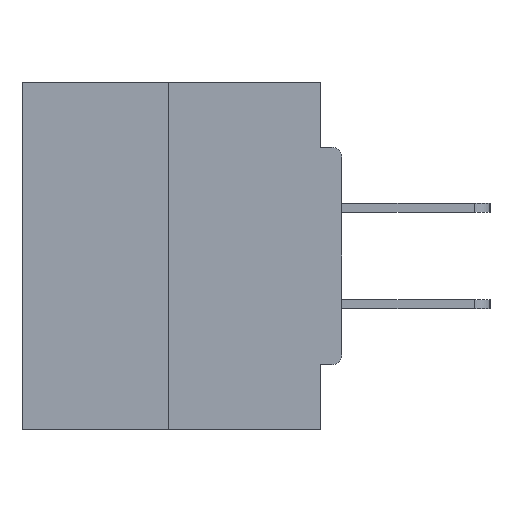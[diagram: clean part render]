
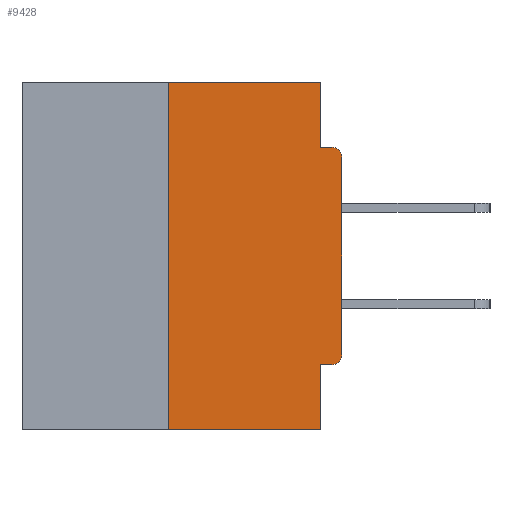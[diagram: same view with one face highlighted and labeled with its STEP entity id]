
A CAD part, left-side view. The second image highlights one B-rep face of the part: STEP entity #9428.
In plain terms, the highlighted planar face has unit normal (-1, 0, 0).
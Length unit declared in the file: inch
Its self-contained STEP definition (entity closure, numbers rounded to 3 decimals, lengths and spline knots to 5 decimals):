
#178 = LINE ( 'NONE', #2677, #25718 ) ;
#254 = PLANE ( 'NONE',  #14358 ) ;
#578 = CARTESIAN_POINT ( 'NONE',  ( 0., 0., -0.1085 ) ) ;
#690 = DIRECTION ( 'NONE',  ( 0., -1., 0. ) ) ;
#1343 = ORIENTED_EDGE ( 'NONE', *, *, #20671, .T. ) ;
#1772 = EDGE_CURVE ( 'NONE', #17126, #13864, #31024, .T. ) ;
#2656 = VECTOR ( 'NONE', #16002, 39.37008 ) ;
#2677 = CARTESIAN_POINT ( 'NONE',  ( 0., 0., -0.4065 ) ) ;
#2802 = VECTOR ( 'NONE', #17738, 39.37008 ) ;
#4215 = DIRECTION ( 'NONE',  ( 1., 0., 0. ) ) ;
#4961 = EDGE_CURVE ( 'NONE', #32058, #18116, #178, .T. ) ;
#5368 = VERTEX_POINT ( 'NONE', #33887 ) ;
#5515 = VERTEX_POINT ( 'NONE', #578 ) ;
#6188 = DIRECTION ( 'NONE',  ( 0., -1., 0. ) ) ;
#6482 = DIRECTION ( 'NONE',  ( 0., 0., -1. ) ) ;
#6739 = CARTESIAN_POINT ( 'NONE',  ( 0., 0.031, -0.5 ) ) ;
#7524 = LINE ( 'NONE', #21823, #31337 ) ;
#8227 = ORIENTED_EDGE ( 'NONE', *, *, #1772, .F. ) ;
#8964 = CARTESIAN_POINT ( 'NONE',  ( 0., 0.015, -0.1085 ) ) ;
#9094 = CARTESIAN_POINT ( 'NONE',  ( 0., 0., -0.0935 ) ) ;
#9354 = EDGE_CURVE ( 'NONE', #13864, #20374, #30465, .T. ) ;
#9428 = ADVANCED_FACE ( 'NONE', ( #26190 ), #254, .F. ) ;
#9786 = ORIENTED_EDGE ( 'NONE', *, *, #19300, .T. ) ;
#10267 = ORIENTED_EDGE ( 'NONE', *, *, #32802, .T. ) ;
#10586 = CARTESIAN_POINT ( 'NONE',  ( 0., 0.25, -0.5 ) ) ;
#10591 = VECTOR ( 'NONE', #6188, 39.37008 ) ;
#10795 = CIRCLE ( 'NONE', #32243, 0.015 ) ;
#11548 = LINE ( 'NONE', #18531, #13664 ) ;
#11606 = DIRECTION ( 'NONE',  ( 0., -1., 0. ) ) ;
#13664 = VECTOR ( 'NONE', #32955, 39.37008 ) ;
#13775 = CARTESIAN_POINT ( 'NONE',  ( 0., 0.25, 0. ) ) ;
#13864 = VERTEX_POINT ( 'NONE', #21802 ) ;
#14011 = CARTESIAN_POINT ( 'NONE',  ( 0., 0.015, -0.3915 ) ) ;
#14358 = AXIS2_PLACEMENT_3D ( 'NONE', #32922, #4215, #6482 ) ;
#14621 = EDGE_LOOP ( 'NONE', ( #8227, #24536, #34592, #26062, #24534, #9786, #1343, #10267, #15903, #28157 ) ) ;
#15578 = VERTEX_POINT ( 'NONE', #10586 ) ;
#15903 = ORIENTED_EDGE ( 'NONE', *, *, #22253, .F. ) ;
#16002 = DIRECTION ( 'NONE',  ( 0., 0., 1. ) ) ;
#16354 = CARTESIAN_POINT ( 'NONE',  ( 0., 0.25, 0. ) ) ;
#16833 = EDGE_CURVE ( 'NONE', #15578, #17126, #29869, .T. ) ;
#17126 = VERTEX_POINT ( 'NONE', #13775 ) ;
#17738 = DIRECTION ( 'NONE',  ( 0., 0., -1. ) ) ;
#18116 = VERTEX_POINT ( 'NONE', #33922 ) ;
#18531 = CARTESIAN_POINT ( 'NONE',  ( 0., 0., 0. ) ) ;
#19300 = EDGE_CURVE ( 'NONE', #32058, #5368, #10795, .T. ) ;
#19548 = CARTESIAN_POINT ( 'NONE',  ( 0., 0.015, -0.4065 ) ) ;
#19780 = CARTESIAN_POINT ( 'NONE',  ( 0., 0.46, 0. ) ) ;
#20374 = VERTEX_POINT ( 'NONE', #23149 ) ;
#20671 = EDGE_CURVE ( 'NONE', #5368, #5515, #11548, .T. ) ;
#21745 = DIRECTION ( 'NONE',  ( 0., 1., 0. ) ) ;
#21802 = CARTESIAN_POINT ( 'NONE',  ( 0., 0.031, 0. ) ) ;
#21823 = CARTESIAN_POINT ( 'NONE',  ( 0., 0.031, -0.5 ) ) ;
#22253 = EDGE_CURVE ( 'NONE', #20374, #32228, #28011, .T. ) ;
#22376 = CARTESIAN_POINT ( 'NONE',  ( 0., 0.46, -0.5 ) ) ;
#22562 = DIRECTION ( 'NONE',  ( 0., 0., -1. ) ) ;
#22721 = EDGE_CURVE ( 'NONE', #18116, #33283, #7524, .T. ) ;
#23149 = CARTESIAN_POINT ( 'NONE',  ( 0., 0.031, -0.0935 ) ) ;
#23221 = EDGE_CURVE ( 'NONE', #15578, #33283, #33869, .T. ) ;
#24534 = ORIENTED_EDGE ( 'NONE', *, *, #4961, .F. ) ;
#24536 = ORIENTED_EDGE ( 'NONE', *, *, #16833, .F. ) ;
#25058 = VECTOR ( 'NONE', #11606, 39.37008 ) ;
#25718 = VECTOR ( 'NONE', #21745, 39.37008 ) ;
#25752 = CIRCLE ( 'NONE', #32561, 0.015 ) ;
#26062 = ORIENTED_EDGE ( 'NONE', *, *, #22721, .F. ) ;
#26190 = FACE_OUTER_BOUND ( 'NONE', #14621, .T. ) ;
#26635 = DIRECTION ( 'NONE',  ( 0., 0., -1. ) ) ;
#28011 = LINE ( 'NONE', #9094, #25058 ) ;
#28157 = ORIENTED_EDGE ( 'NONE', *, *, #9354, .F. ) ;
#29869 = LINE ( 'NONE', #16354, #2656 ) ;
#30343 = DIRECTION ( 'NONE',  ( -1., 0., 0. ) ) ;
#30465 = LINE ( 'NONE', #31979, #2802 ) ;
#30718 = DIRECTION ( 'NONE',  ( 0., 0., -1. ) ) ;
#31024 = LINE ( 'NONE', #19780, #10591 ) ;
#31337 = VECTOR ( 'NONE', #26635, 39.37008 ) ;
#31735 = CARTESIAN_POINT ( 'NONE',  ( 0., 0.015, -0.0935 ) ) ;
#31979 = CARTESIAN_POINT ( 'NONE',  ( 0., 0.031, 0. ) ) ;
#32058 = VERTEX_POINT ( 'NONE', #19548 ) ;
#32228 = VERTEX_POINT ( 'NONE', #31735 ) ;
#32243 = AXIS2_PLACEMENT_3D ( 'NONE', #14011, #32968, #30718 ) ;
#32561 = AXIS2_PLACEMENT_3D ( 'NONE', #8964, #30343, #22562 ) ;
#32576 = VECTOR ( 'NONE', #690, 39.37008 ) ;
#32802 = EDGE_CURVE ( 'NONE', #5515, #32228, #25752, .T. ) ;
#32922 = CARTESIAN_POINT ( 'NONE',  ( 0., 0.46, 0. ) ) ;
#32955 = DIRECTION ( 'NONE',  ( 0., 0., 1. ) ) ;
#32968 = DIRECTION ( 'NONE',  ( -1., 0., 0. ) ) ;
#33283 = VERTEX_POINT ( 'NONE', #6739 ) ;
#33869 = LINE ( 'NONE', #22376, #32576 ) ;
#33887 = CARTESIAN_POINT ( 'NONE',  ( 0., 0., -0.3915 ) ) ;
#33922 = CARTESIAN_POINT ( 'NONE',  ( 0., 0.031, -0.4065 ) ) ;
#34592 = ORIENTED_EDGE ( 'NONE', *, *, #23221, .T. ) ;
